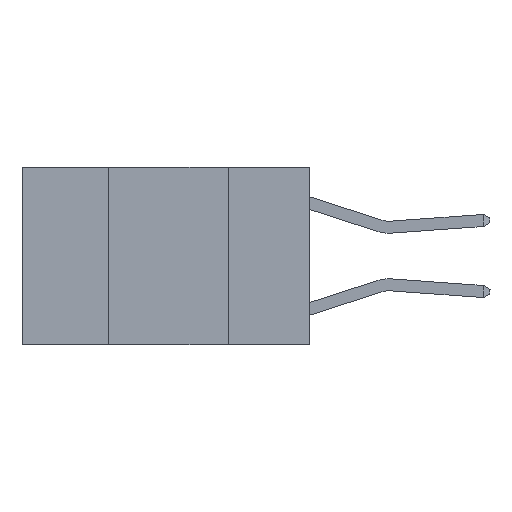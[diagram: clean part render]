
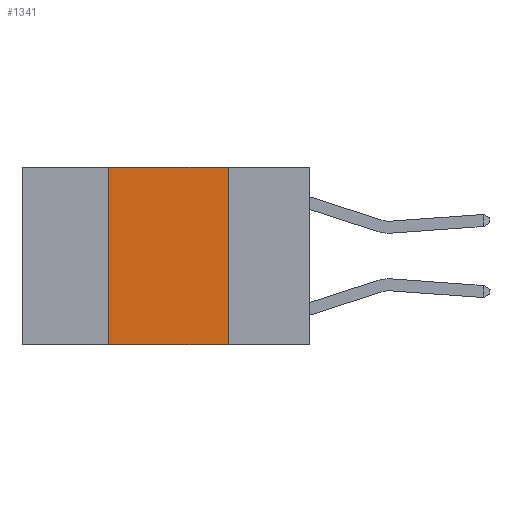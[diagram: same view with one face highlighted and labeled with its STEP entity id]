
A CAD part, left-side view. The second image highlights one B-rep face of the part: STEP entity #1341.
In plain terms, the highlighted planar face has unit normal (-1, 0, 0).
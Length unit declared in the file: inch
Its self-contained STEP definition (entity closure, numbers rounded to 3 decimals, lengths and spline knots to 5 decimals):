
#776 = VECTOR ( 'NONE', #8317, 39.37008 ) ;
#785 = PLANE ( 'NONE',  #4285 ) ;
#1178 = LINE ( 'NONE', #5759, #776 ) ;
#1341 = ADVANCED_FACE ( 'NONE', ( #12913 ), #785, .F. ) ;
#1509 = ORIENTED_EDGE ( 'NONE', *, *, #16158, .F. ) ;
#2422 = CARTESIAN_POINT ( 'NONE',  ( 0., 0.42, 0. ) ) ;
#2480 = CARTESIAN_POINT ( 'NONE',  ( 0., 0.42, -0.37 ) ) ;
#3321 = DIRECTION ( 'NONE',  ( 0., 0., -1. ) ) ;
#4081 = VECTOR ( 'NONE', #11428, 39.37008 ) ;
#4188 = VERTEX_POINT ( 'NONE', #11484 ) ;
#4285 = AXIS2_PLACEMENT_3D ( 'NONE', #9656, #10933, #3321 ) ;
#4884 = LINE ( 'NONE', #12652, #4081 ) ;
#4963 = EDGE_LOOP ( 'NONE', ( #13574, #10979, #1509, #15010 ) ) ;
#5661 = LINE ( 'NONE', #10023, #11236 ) ;
#5759 = CARTESIAN_POINT ( 'NONE',  ( 0., 0.42, 0. ) ) ;
#5833 = VECTOR ( 'NONE', #7461, 39.37008 ) ;
#6382 = CARTESIAN_POINT ( 'NONE',  ( 0., 0.17, 0. ) ) ;
#7461 = DIRECTION ( 'NONE',  ( 0., -1., 0. ) ) ;
#8317 = DIRECTION ( 'NONE',  ( 0., 0., 1. ) ) ;
#8569 = EDGE_CURVE ( 'NONE', #13728, #15789, #5661, .T. ) ;
#8610 = EDGE_CURVE ( 'NONE', #15789, #4188, #4884, .T. ) ;
#8821 = LINE ( 'NONE', #15055, #5833 ) ;
#9173 = EDGE_CURVE ( 'NONE', #11343, #4188, #8821, .T. ) ;
#9656 = CARTESIAN_POINT ( 'NONE',  ( 0., 0.6, 0. ) ) ;
#10023 = CARTESIAN_POINT ( 'NONE',  ( 0., 0.6, 0. ) ) ;
#10933 = DIRECTION ( 'NONE',  ( 1., 0., 0. ) ) ;
#10979 = ORIENTED_EDGE ( 'NONE', *, *, #8569, .F. ) ;
#11236 = VECTOR ( 'NONE', #13863, 39.37008 ) ;
#11343 = VERTEX_POINT ( 'NONE', #2480 ) ;
#11428 = DIRECTION ( 'NONE',  ( 0., 0., -1. ) ) ;
#11484 = CARTESIAN_POINT ( 'NONE',  ( 0., 0.17, -0.37 ) ) ;
#12652 = CARTESIAN_POINT ( 'NONE',  ( 0., 0.17, 0. ) ) ;
#12913 = FACE_OUTER_BOUND ( 'NONE', #4963, .T. ) ;
#13574 = ORIENTED_EDGE ( 'NONE', *, *, #8610, .F. ) ;
#13728 = VERTEX_POINT ( 'NONE', #2422 ) ;
#13863 = DIRECTION ( 'NONE',  ( 0., -1., 0. ) ) ;
#15010 = ORIENTED_EDGE ( 'NONE', *, *, #9173, .T. ) ;
#15055 = CARTESIAN_POINT ( 'NONE',  ( 0., 0.6, -0.37 ) ) ;
#15789 = VERTEX_POINT ( 'NONE', #6382 ) ;
#16158 = EDGE_CURVE ( 'NONE', #11343, #13728, #1178, .T. ) ;
